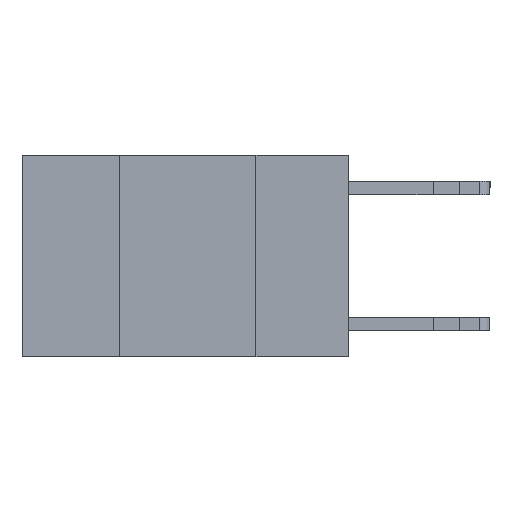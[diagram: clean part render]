
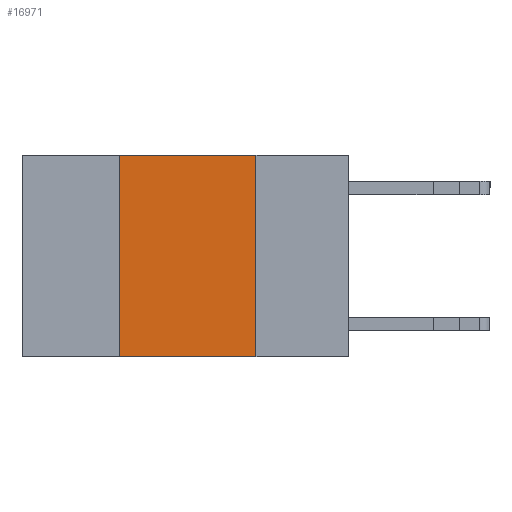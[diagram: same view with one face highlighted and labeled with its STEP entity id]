
A CAD part, left-side view. The second image highlights one B-rep face of the part: STEP entity #16971.
In plain terms, the highlighted planar face has unit normal (-1, 0, 0).
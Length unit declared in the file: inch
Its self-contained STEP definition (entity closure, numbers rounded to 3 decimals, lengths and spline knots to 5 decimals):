
#482 = CARTESIAN_POINT ( 'NONE',  ( 0., 0.42, -0.37 ) ) ;
#874 = DIRECTION ( 'NONE',  ( 0., 0., -1. ) ) ;
#1063 = CARTESIAN_POINT ( 'NONE',  ( 0., 0.6, 0. ) ) ;
#1115 = LINE ( 'NONE', #7111, #17066 ) ;
#3800 = CARTESIAN_POINT ( 'NONE',  ( 0., 0.42, 0. ) ) ;
#3840 = CARTESIAN_POINT ( 'NONE',  ( 0., 0.17, -0.37 ) ) ;
#4228 = EDGE_LOOP ( 'NONE', ( #16857, #7093, #17616, #13147 ) ) ;
#5603 = LINE ( 'NONE', #7054, #9328 ) ;
#5855 = DIRECTION ( 'NONE',  ( 0., -1., 0. ) ) ;
#6092 = EDGE_CURVE ( 'NONE', #13670, #6463, #17192, .T. ) ;
#6463 = VERTEX_POINT ( 'NONE', #10624 ) ;
#6708 = VECTOR ( 'NONE', #6883, 39.37008 ) ;
#6883 = DIRECTION ( 'NONE',  ( 0., -1., 0. ) ) ;
#7054 = CARTESIAN_POINT ( 'NONE',  ( 0., 0.17, 0. ) ) ;
#7093 = ORIENTED_EDGE ( 'NONE', *, *, #6092, .F. ) ;
#7111 = CARTESIAN_POINT ( 'NONE',  ( 0., 0.6, -0.37 ) ) ;
#7676 = VECTOR ( 'NONE', #14340, 39.37008 ) ;
#8510 = DIRECTION ( 'NONE',  ( 0., 0., -1. ) ) ;
#8960 = VERTEX_POINT ( 'NONE', #482 ) ;
#9328 = VECTOR ( 'NONE', #874, 39.37008 ) ;
#9885 = LINE ( 'NONE', #9981, #7676 ) ;
#9981 = CARTESIAN_POINT ( 'NONE',  ( 0., 0.42, 0. ) ) ;
#10624 = CARTESIAN_POINT ( 'NONE',  ( 0., 0.17, 0. ) ) ;
#11393 = FACE_OUTER_BOUND ( 'NONE', #4228, .T. ) ;
#11822 = VERTEX_POINT ( 'NONE', #3840 ) ;
#12425 = AXIS2_PLACEMENT_3D ( 'NONE', #1063, #14306, #8510 ) ;
#13147 = ORIENTED_EDGE ( 'NONE', *, *, #18482, .T. ) ;
#13209 = EDGE_CURVE ( 'NONE', #8960, #13670, #9885, .T. ) ;
#13670 = VERTEX_POINT ( 'NONE', #3800 ) ;
#14218 = PLANE ( 'NONE',  #12425 ) ;
#14306 = DIRECTION ( 'NONE',  ( 1., 0., 0. ) ) ;
#14340 = DIRECTION ( 'NONE',  ( 0., 0., 1. ) ) ;
#16857 = ORIENTED_EDGE ( 'NONE', *, *, #16881, .F. ) ;
#16881 = EDGE_CURVE ( 'NONE', #6463, #11822, #5603, .T. ) ;
#16971 = ADVANCED_FACE ( 'NONE', ( #11393 ), #14218, .F. ) ;
#17066 = VECTOR ( 'NONE', #5855, 39.37008 ) ;
#17192 = LINE ( 'NONE', #18751, #6708 ) ;
#17616 = ORIENTED_EDGE ( 'NONE', *, *, #13209, .F. ) ;
#18482 = EDGE_CURVE ( 'NONE', #8960, #11822, #1115, .T. ) ;
#18751 = CARTESIAN_POINT ( 'NONE',  ( 0., 0.6, 0. ) ) ;
